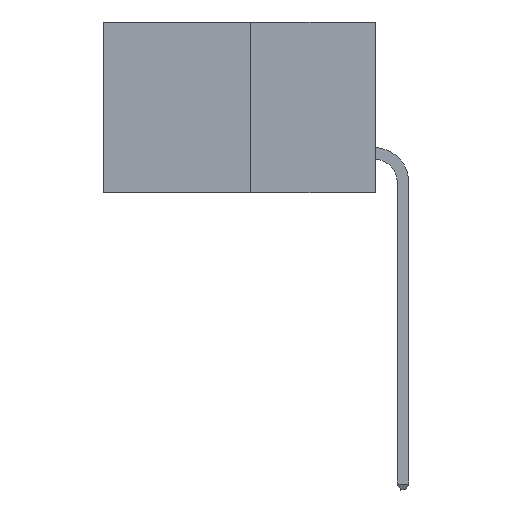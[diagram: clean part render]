
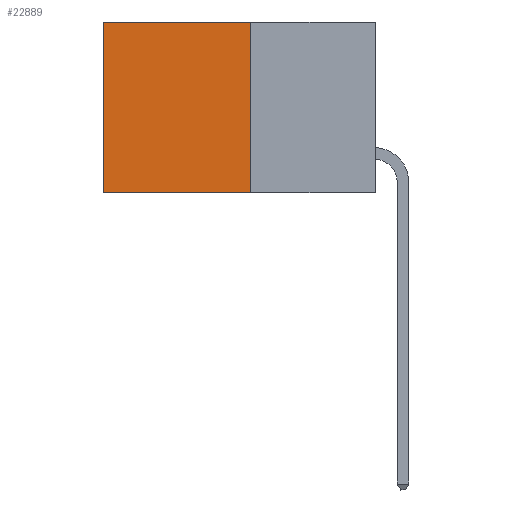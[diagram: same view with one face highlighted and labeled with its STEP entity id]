
A CAD part, left-side view. The second image highlights one B-rep face of the part: STEP entity #22889.
In plain terms, the highlighted planar face has unit normal (-1, 0, 0).
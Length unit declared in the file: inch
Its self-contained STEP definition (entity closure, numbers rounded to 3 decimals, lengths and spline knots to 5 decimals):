
#2653 = VECTOR ( 'NONE', #21982, 39.37008 ) ;
#2848 = EDGE_CURVE ( 'NONE', #14733, #10849, #16119, .T. ) ;
#3993 = CARTESIAN_POINT ( 'NONE',  ( 0.277, 0.59, -0.37 ) ) ;
#4586 = LINE ( 'NONE', #9139, #26660 ) ;
#4698 = EDGE_LOOP ( 'NONE', ( #14722, #23480, #21565, #25388 ) ) ;
#4944 = VECTOR ( 'NONE', #18615, 39.37008 ) ;
#7024 = CARTESIAN_POINT ( 'NONE',  ( 0.277, 0.27, 0. ) ) ;
#7427 = CARTESIAN_POINT ( 'NONE',  ( 0.277, 0.27, -0.37 ) ) ;
#7754 = VECTOR ( 'NONE', #26338, 39.37008 ) ;
#9139 = CARTESIAN_POINT ( 'NONE',  ( 0.277, 0.27, 0. ) ) ;
#9616 = PLANE ( 'NONE',  #9823 ) ;
#9823 = AXIS2_PLACEMENT_3D ( 'NONE', #7427, #11742, #26203 ) ;
#9921 = VERTEX_POINT ( 'NONE', #7024 ) ;
#10849 = VERTEX_POINT ( 'NONE', #20335 ) ;
#11472 = CARTESIAN_POINT ( 'NONE',  ( 0.277, 0.27, -0.37 ) ) ;
#11742 = DIRECTION ( 'NONE',  ( 1., 0., 0. ) ) ;
#14722 = ORIENTED_EDGE ( 'NONE', *, *, #2848, .T. ) ;
#14733 = VERTEX_POINT ( 'NONE', #24952 ) ;
#14940 = EDGE_CURVE ( 'NONE', #9921, #14733, #4586, .T. ) ;
#16119 = LINE ( 'NONE', #3993, #4944 ) ;
#17917 = CARTESIAN_POINT ( 'NONE',  ( 0.277, 0.27, -0.37 ) ) ;
#18615 = DIRECTION ( 'NONE',  ( 0., 0., -1. ) ) ;
#18958 = FACE_OUTER_BOUND ( 'NONE', #4698, .T. ) ;
#20335 = CARTESIAN_POINT ( 'NONE',  ( 0.277, 0.59, -0.37 ) ) ;
#21565 = ORIENTED_EDGE ( 'NONE', *, *, #26417, .F. ) ;
#21982 = DIRECTION ( 'NONE',  ( 0., 1., 0. ) ) ;
#22145 = EDGE_CURVE ( 'NONE', #25153, #10849, #24782, .T. ) ;
#22889 = ADVANCED_FACE ( 'NONE', ( #18958 ), #9616, .F. ) ;
#23480 = ORIENTED_EDGE ( 'NONE', *, *, #22145, .F. ) ;
#23746 = DIRECTION ( 'NONE',  ( 0., 1., 0. ) ) ;
#24324 = CARTESIAN_POINT ( 'NONE',  ( 0.277, 0.27, -0.37 ) ) ;
#24380 = LINE ( 'NONE', #24324, #7754 ) ;
#24782 = LINE ( 'NONE', #17917, #2653 ) ;
#24952 = CARTESIAN_POINT ( 'NONE',  ( 0.277, 0.59, 0. ) ) ;
#25153 = VERTEX_POINT ( 'NONE', #11472 ) ;
#25388 = ORIENTED_EDGE ( 'NONE', *, *, #14940, .T. ) ;
#26203 = DIRECTION ( 'NONE',  ( 0., 0., -1. ) ) ;
#26338 = DIRECTION ( 'NONE',  ( 0., 0., -1. ) ) ;
#26417 = EDGE_CURVE ( 'NONE', #9921, #25153, #24380, .T. ) ;
#26660 = VECTOR ( 'NONE', #23746, 39.37008 ) ;
